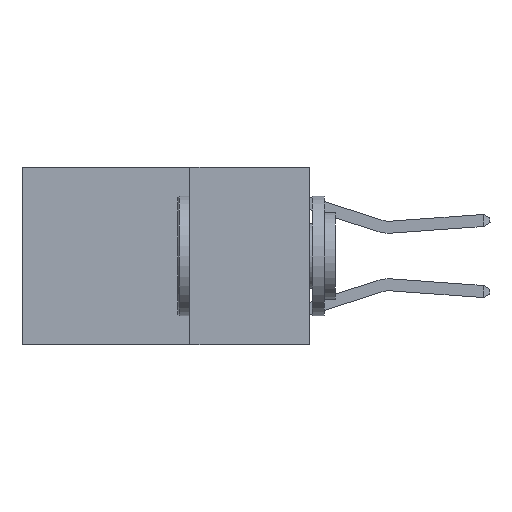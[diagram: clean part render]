
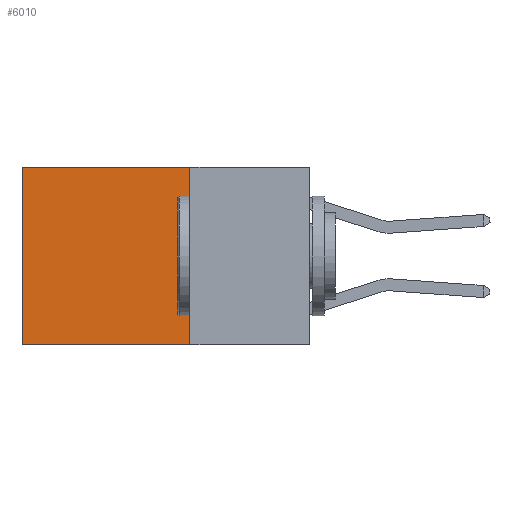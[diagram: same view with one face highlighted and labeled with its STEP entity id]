
A CAD part, left-side view. The second image highlights one B-rep face of the part: STEP entity #6010.
In plain terms, the highlighted planar face has unit normal (-1, 0, 0).
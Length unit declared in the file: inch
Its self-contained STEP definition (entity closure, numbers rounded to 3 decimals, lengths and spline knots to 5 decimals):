
#847 = CARTESIAN_POINT ( 'NONE',  ( 0.2625, 0.6, 0. ) ) ;
#1015 = VECTOR ( 'NONE', #7814, 39.37008 ) ;
#1130 = ORIENTED_EDGE ( 'NONE', *, *, #8716, .T. ) ;
#1386 = EDGE_LOOP ( 'NONE', ( #10701, #2369, #2117, #1130 ) ) ;
#1392 = AXIS2_PLACEMENT_3D ( 'NONE', #2625, #9986, #5269 ) ;
#1881 = DIRECTION ( 'NONE',  ( 0., 0., -1. ) ) ;
#2117 = ORIENTED_EDGE ( 'NONE', *, *, #8914, .F. ) ;
#2131 = VERTEX_POINT ( 'NONE', #847 ) ;
#2338 = FACE_OUTER_BOUND ( 'NONE', #1386, .T. ) ;
#2369 = ORIENTED_EDGE ( 'NONE', *, *, #4455, .F. ) ;
#2392 = LINE ( 'NONE', #8543, #6887 ) ;
#2625 = CARTESIAN_POINT ( 'NONE',  ( 0.2625, 0.25, 0. ) ) ;
#2642 = LINE ( 'NONE', #4173, #7092 ) ;
#2782 = VERTEX_POINT ( 'NONE', #5384 ) ;
#2899 = CARTESIAN_POINT ( 'NONE',  ( 0.2625, 0.25, -0.37 ) ) ;
#3376 = VECTOR ( 'NONE', #3488, 39.37008 ) ;
#3488 = DIRECTION ( 'NONE',  ( 0., 0., -1. ) ) ;
#3890 = EDGE_CURVE ( 'NONE', #2131, #4607, #2392, .T. ) ;
#4173 = CARTESIAN_POINT ( 'NONE',  ( 0.2625, 0.25, 0. ) ) ;
#4455 = EDGE_CURVE ( 'NONE', #2782, #4607, #5789, .T. ) ;
#4458 = PLANE ( 'NONE',  #1392 ) ;
#4607 = VERTEX_POINT ( 'NONE', #8163 ) ;
#5269 = DIRECTION ( 'NONE',  ( 0., 0., -1. ) ) ;
#5384 = CARTESIAN_POINT ( 'NONE',  ( 0.2625, 0.25, -0.37 ) ) ;
#5789 = LINE ( 'NONE', #2899, #1015 ) ;
#5905 = LINE ( 'NONE', #7503, #3376 ) ;
#5966 = VERTEX_POINT ( 'NONE', #6035 ) ;
#6010 = ADVANCED_FACE ( 'NONE', ( #2338 ), #4458, .F. ) ;
#6035 = CARTESIAN_POINT ( 'NONE',  ( 0.2625, 0.25, 0. ) ) ;
#6887 = VECTOR ( 'NONE', #1881, 39.37008 ) ;
#7092 = VECTOR ( 'NONE', #9730, 39.37008 ) ;
#7503 = CARTESIAN_POINT ( 'NONE',  ( 0.2625, 0.25, 0. ) ) ;
#7814 = DIRECTION ( 'NONE',  ( 0., 1., 0. ) ) ;
#8163 = CARTESIAN_POINT ( 'NONE',  ( 0.2625, 0.6, -0.37 ) ) ;
#8543 = CARTESIAN_POINT ( 'NONE',  ( 0.2625, 0.6, 0. ) ) ;
#8716 = EDGE_CURVE ( 'NONE', #5966, #2131, #2642, .T. ) ;
#8914 = EDGE_CURVE ( 'NONE', #5966, #2782, #5905, .T. ) ;
#9730 = DIRECTION ( 'NONE',  ( 0., 1., 0. ) ) ;
#9986 = DIRECTION ( 'NONE',  ( 1., 0., 0. ) ) ;
#10701 = ORIENTED_EDGE ( 'NONE', *, *, #3890, .T. ) ;
